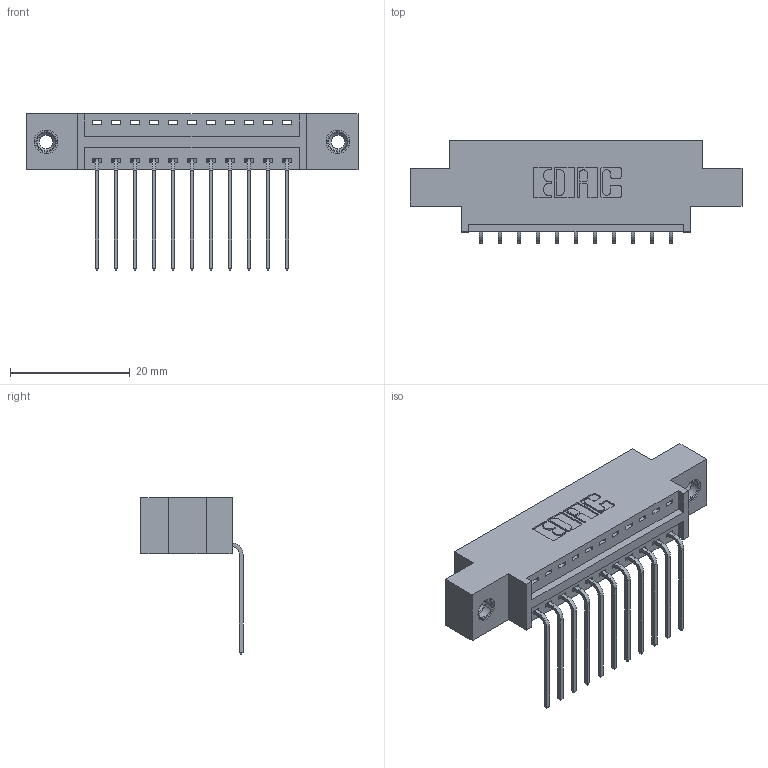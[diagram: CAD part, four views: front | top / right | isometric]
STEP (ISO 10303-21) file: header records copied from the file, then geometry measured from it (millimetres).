
FILE_DESCRIPTION (( 'STEP AP203' ), '1' );
FILE_NAME ('396-011-559-608.STEP', '2019-10-31T20:16:47', ( '' ), ( '' ), 'SwSTEP 2.0', 'SolidWorks 2016', '' );
FILE_SCHEMA (( 'CONFIG_CONTROL_DESIGN' ));
Length unit declared in the file: inch
Products named in the file (4): 346 Part_0.170 Offset - 0.156 Dia-TI; 345-292-001_558 559 Tail - 1; 345-250-001_345-250-003-102; 396-011-559-608
Assembly tree (14 placements, depth 2):
  396-011-559-608
    346 Part_0.170 Offset - 0.156 Dia-TI
    345-292-001_558 559 Tail - 1  x11
    345-250-001_345-250-003-102  x2
Bounding box: 55.5 x 17.08 x 26.16 mm (x, y, z)
Volume: 4974.4 mm3; surface area: 6283.6 mm2
Topology: 14 solids, 14 shells, 846 faces, 2479 edges, 1630 vertices
Faces by surface type: plane 574, cylinder 256, cone 12, torus 4
Entity records: 12402 total; most frequent: CARTESIAN_POINT 2120, ORIENTED_EDGE 2058, DIRECTION 1933, EDGE_CURVE 1029, LINE 833, VECTOR 833, VERTEX_POINT 680, AXIS2_PLACEMENT_3D 550
